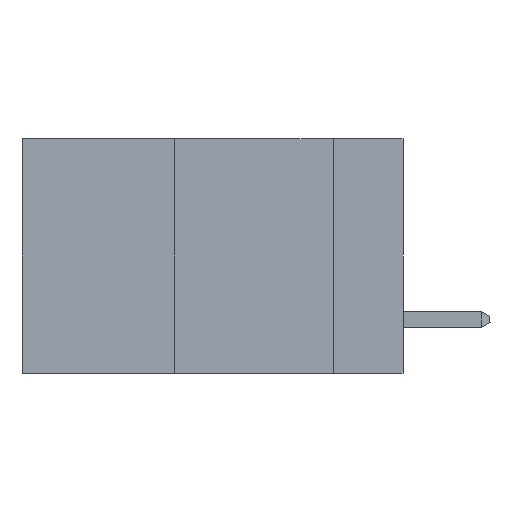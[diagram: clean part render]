
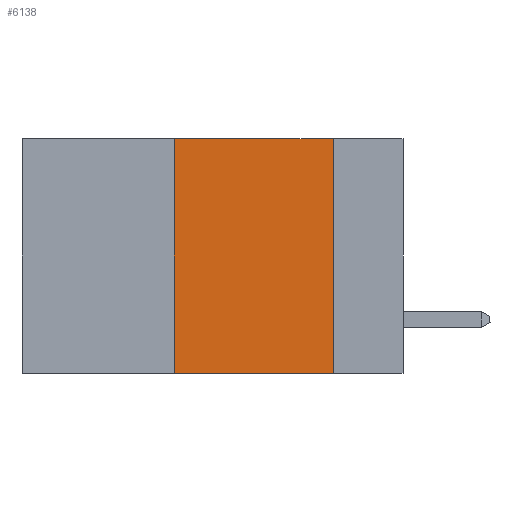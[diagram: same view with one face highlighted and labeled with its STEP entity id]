
A CAD part, left-side view. The second image highlights one B-rep face of the part: STEP entity #6138.
In plain terms, the highlighted planar face has unit normal (-1, 0, 0).
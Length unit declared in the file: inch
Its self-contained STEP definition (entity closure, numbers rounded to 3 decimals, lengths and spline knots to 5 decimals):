
#212 = LINE ( 'NONE', #3682, #9997 ) ;
#784 = CARTESIAN_POINT ( 'NONE',  ( 0., 0.36, 0. ) ) ;
#798 = VERTEX_POINT ( 'NONE', #1549 ) ;
#1140 = VECTOR ( 'NONE', #12926, 39.37008 ) ;
#1236 = EDGE_CURVE ( 'NONE', #1643, #798, #2217, .T. ) ;
#1465 = AXIS2_PLACEMENT_3D ( 'NONE', #10349, #9191, #12111 ) ;
#1549 = CARTESIAN_POINT ( 'NONE',  ( 0., 0.11, 0. ) ) ;
#1643 = VERTEX_POINT ( 'NONE', #10926 ) ;
#2217 = LINE ( 'NONE', #2835, #9994 ) ;
#2835 = CARTESIAN_POINT ( 'NONE',  ( 0., 0.6, 0. ) ) ;
#3206 = ORIENTED_EDGE ( 'NONE', *, *, #3393, .F. ) ;
#3393 = EDGE_CURVE ( 'NONE', #798, #6779, #212, .T. ) ;
#3453 = EDGE_CURVE ( 'NONE', #7246, #6779, #9409, .T. ) ;
#3475 = EDGE_CURVE ( 'NONE', #7246, #1643, #6857, .T. ) ;
#3682 = CARTESIAN_POINT ( 'NONE',  ( 0., 0.11, 0. ) ) ;
#4025 = CARTESIAN_POINT ( 'NONE',  ( 0., 0.6, -0.37 ) ) ;
#4056 = VECTOR ( 'NONE', #12001, 39.37008 ) ;
#4582 = ORIENTED_EDGE ( 'NONE', *, *, #1236, .F. ) ;
#4772 = DIRECTION ( 'NONE',  ( 0., 0., -1. ) ) ;
#5574 = CARTESIAN_POINT ( 'NONE',  ( 0., 0.36, -0.37 ) ) ;
#6138 = ADVANCED_FACE ( 'NONE', ( #9795 ), #8015, .F. ) ;
#6590 = ORIENTED_EDGE ( 'NONE', *, *, #3453, .T. ) ;
#6779 = VERTEX_POINT ( 'NONE', #7032 ) ;
#6857 = LINE ( 'NONE', #784, #4056 ) ;
#7032 = CARTESIAN_POINT ( 'NONE',  ( 0., 0.11, -0.37 ) ) ;
#7090 = DIRECTION ( 'NONE',  ( 0., -1., 0. ) ) ;
#7246 = VERTEX_POINT ( 'NONE', #5574 ) ;
#7349 = EDGE_LOOP ( 'NONE', ( #3206, #4582, #12357, #6590 ) ) ;
#8015 = PLANE ( 'NONE',  #1465 ) ;
#9191 = DIRECTION ( 'NONE',  ( 1., 0., 0. ) ) ;
#9409 = LINE ( 'NONE', #4025, #1140 ) ;
#9795 = FACE_OUTER_BOUND ( 'NONE', #7349, .T. ) ;
#9994 = VECTOR ( 'NONE', #7090, 39.37008 ) ;
#9997 = VECTOR ( 'NONE', #4772, 39.37008 ) ;
#10349 = CARTESIAN_POINT ( 'NONE',  ( 0., 0.6, 0. ) ) ;
#10926 = CARTESIAN_POINT ( 'NONE',  ( 0., 0.36, 0. ) ) ;
#12001 = DIRECTION ( 'NONE',  ( 0., 0., 1. ) ) ;
#12111 = DIRECTION ( 'NONE',  ( 0., 0., -1. ) ) ;
#12357 = ORIENTED_EDGE ( 'NONE', *, *, #3475, .F. ) ;
#12926 = DIRECTION ( 'NONE',  ( 0., -1., 0. ) ) ;
